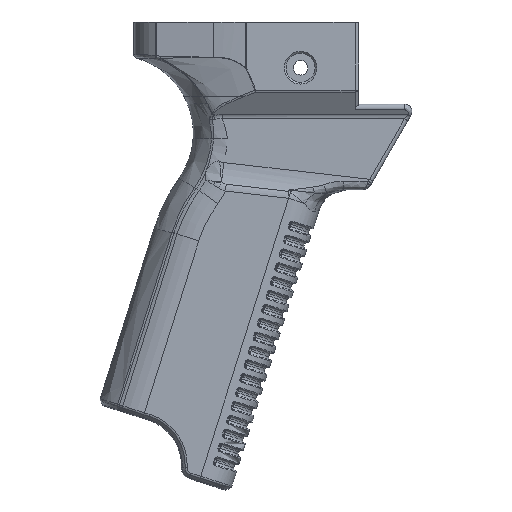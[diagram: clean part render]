
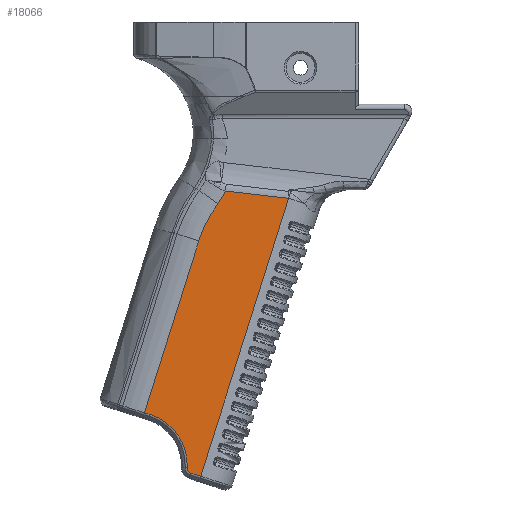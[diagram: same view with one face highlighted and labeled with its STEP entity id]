
A CAD part, front view. The second image highlights one B-rep face of the part: STEP entity #18066.
In plain terms, the highlighted planar face has unit normal (0, -1, 0).
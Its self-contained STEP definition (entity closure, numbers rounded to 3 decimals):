
#251=PLANE('',#19877);
#398=LINE('',#25994,#1295);
#911=LINE('',#37858,#1808);
#912=LINE('',#37869,#1809);
#956=LINE('',#38597,#1853);
#957=LINE('',#38606,#1854);
#1295=VECTOR('',#20653,10.);
#1808=VECTOR('',#23696,10.);
#1809=VECTOR('',#23713,10.);
#1853=VECTOR('',#23953,10.);
#1854=VECTOR('',#23958,10.);
#2978=B_SPLINE_CURVE_WITH_KNOTS('',3,(#38601,#38602,#38603,#38604),
 .UNSPECIFIED.,.F.,.F.,(4,4),(-0.018,0.),
 .UNSPECIFIED.);
#4371=FACE_OUTER_BOUND('',#5563,.T.);
#5563=EDGE_LOOP('',(#15163,#15164,#15165,#15166,#15167,#15168,#15169,#15170,
#15171,#15172));
#6710=CIRCLE('',#19772,14.581);
#6712=CIRCLE('',#19775,1.419);
#6767=CIRCLE('',#19878,34.246);
#6768=CIRCLE('',#19879,37.23);
#7212=VERTEX_POINT('',#25988);
#7213=VERTEX_POINT('',#25993);
#8105=VERTEX_POINT('',#37849);
#8106=VERTEX_POINT('',#37856);
#8107=VERTEX_POINT('',#37860);
#8108=VERTEX_POINT('',#37864);
#8168=VERTEX_POINT('',#38596);
#8169=VERTEX_POINT('',#38600);
#8170=VERTEX_POINT('',#38605);
#8171=VERTEX_POINT('',#38607);
#8822=EDGE_CURVE('',#7212,#7213,#398,.T.);
#10474=EDGE_CURVE('',#8106,#8105,#911,.T.);
#10476=EDGE_CURVE('',#8107,#8106,#6710,.T.);
#10478=EDGE_CURVE('',#8108,#8107,#6712,.T.);
#10480=EDGE_CURVE('',#7213,#8108,#912,.T.);
#10599=EDGE_CURVE('',#8105,#8168,#956,.T.);
#10601=EDGE_CURVE('',#8169,#7212,#2978,.T.);
#10602=EDGE_CURVE('',#8170,#8169,#957,.T.);
#10603=EDGE_CURVE('',#8171,#8170,#6767,.T.);
#10604=EDGE_CURVE('',#8168,#8171,#6768,.T.);
#15163=ORIENTED_EDGE('',*,*,#8822,.F.);
#15164=ORIENTED_EDGE('',*,*,#10601,.F.);
#15165=ORIENTED_EDGE('',*,*,#10602,.F.);
#15166=ORIENTED_EDGE('',*,*,#10603,.F.);
#15167=ORIENTED_EDGE('',*,*,#10604,.F.);
#15168=ORIENTED_EDGE('',*,*,#10599,.F.);
#15169=ORIENTED_EDGE('',*,*,#10474,.F.);
#15170=ORIENTED_EDGE('',*,*,#10476,.F.);
#15171=ORIENTED_EDGE('',*,*,#10478,.F.);
#15172=ORIENTED_EDGE('',*,*,#10480,.F.);
#18066=ADVANCED_FACE('',(#4371),#251,.T.);
#19772=AXIS2_PLACEMENT_3D('',#37862,#23701,#23702);
#19775=AXIS2_PLACEMENT_3D('',#37866,#23707,#23708);
#19877=AXIS2_PLACEMENT_3D('',#38599,#23956,#23957);
#19878=AXIS2_PLACEMENT_3D('',#38608,#23959,#23960);
#19879=AXIS2_PLACEMENT_3D('',#38609,#23961,#23962);
#20653=DIRECTION('',(-0.301,0.,-0.953));
#23696=DIRECTION('',(-0.953,0.,0.301));
#23701=DIRECTION('center_axis',(0.,-1.,0.));
#23702=DIRECTION('ref_axis',(0.822,0.,0.569));
#23707=DIRECTION('center_axis',(0.,1.,0.));
#23708=DIRECTION('ref_axis',(-0.822,0.,-0.569));
#23713=DIRECTION('',(-0.953,0.,0.301));
#23953=DIRECTION('',(0.301,0.,0.953));
#23956=DIRECTION('center_axis',(0.,-1.,0.));
#23957=DIRECTION('ref_axis',(1.,0.,0.));
#23958=DIRECTION('',(0.993,0.,-0.114));
#23959=DIRECTION('center_axis',(0.,-1.,0.));
#23960=DIRECTION('ref_axis',(0.833,0.,-0.553));
#23961=DIRECTION('center_axis',(0.,1.,0.));
#23962=DIRECTION('ref_axis',(-0.888,0.,0.459));
#25988=CARTESIAN_POINT('',(-154.447,3.068,-51.022));
#25993=CARTESIAN_POINT('',(-178.613,3.068,-127.473));
#25994=CARTESIAN_POINT('',(-158.165,3.068,-62.785));
#37849=CARTESIAN_POINT('',(-194.075,3.068,-110.));
#37856=CARTESIAN_POINT('',(-192.507,3.068,-110.496));
#37858=CARTESIAN_POINT('',(-174.614,3.068,-116.151));
#37860=CARTESIAN_POINT('',(-182.341,3.068,-125.178));
#37862=CARTESIAN_POINT('Origin',(-196.901,3.068,-124.399));
#37864=CARTESIAN_POINT('',(-181.352,3.068,-126.607));
#37866=CARTESIAN_POINT('Origin',(-180.924,3.068,-125.254));
#37869=CARTESIAN_POINT('',(-176.104,3.068,-128.266));
#38596=CARTESIAN_POINT('',(-179.14,3.068,-62.751));
#38597=CARTESIAN_POINT('',(-179.058,3.068,-62.491));
#38599=CARTESIAN_POINT('Origin',(-159.401,3.068,-74.198));
#38600=CARTESIAN_POINT('',(-154.624,3.068,-50.984));
#38601=CARTESIAN_POINT('Ctrl Pts',(-154.624,3.068,-50.984));
#38602=CARTESIAN_POINT('Ctrl Pts',(-154.564,3.068,-50.991));
#38603=CARTESIAN_POINT('Ctrl Pts',(-154.505,3.068,-51.003));
#38604=CARTESIAN_POINT('Ctrl Pts',(-154.447,3.068,-51.022));
#38605=CARTESIAN_POINT('',(-171.8,3.068,-49.012));
#38606=CARTESIAN_POINT('',(-144.123,3.068,-52.19));
#38607=CARTESIAN_POINT('',(-173.881,3.068,-52.467));
#38608=CARTESIAN_POINT('Origin',(-202.126,3.068,-33.103));
#38609=CARTESIAN_POINT('Origin',(-143.765,3.068,-74.355));
